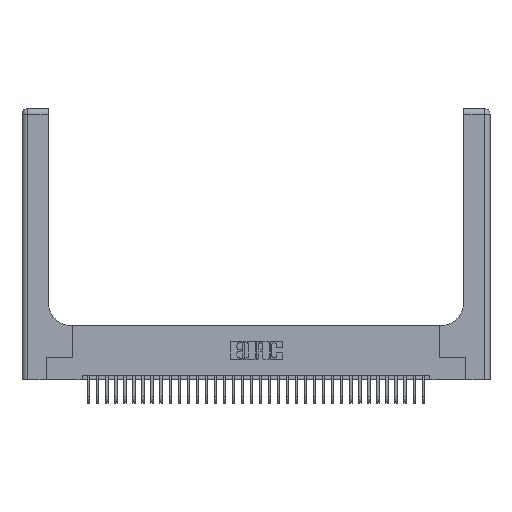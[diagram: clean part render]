
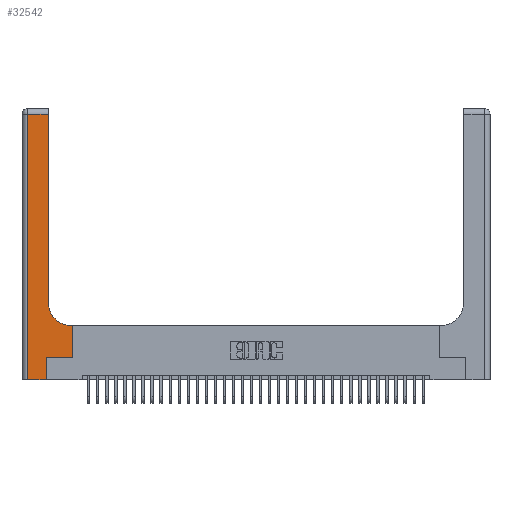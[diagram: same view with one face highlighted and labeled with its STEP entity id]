
A CAD part, top view. The second image highlights one B-rep face of the part: STEP entity #32542.
In plain terms, the highlighted planar face has unit normal (0, 0, 1).
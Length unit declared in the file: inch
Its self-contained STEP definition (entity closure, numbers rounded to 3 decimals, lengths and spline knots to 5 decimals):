
#166 = DIRECTION ( 'NONE',  ( 0., -1., 0. ) ) ;
#376 = VERTEX_POINT ( 'NONE', #32147 ) ;
#468 = CIRCLE ( 'NONE', #10036, 0.25 ) ;
#1016 = VERTEX_POINT ( 'NONE', #6161 ) ;
#1091 = CARTESIAN_POINT ( 'NONE',  ( 0., 3., 0.37 ) ) ;
#1142 = ORIENTED_EDGE ( 'NONE', *, *, #17522, .T. ) ;
#2170 = CARTESIAN_POINT ( 'NONE',  ( 0.5585, 0.25, 0.37 ) ) ;
#2455 = ORIENTED_EDGE ( 'NONE', *, *, #17761, .T. ) ;
#2585 = LINE ( 'NONE', #32829, #16213 ) ;
#3007 = EDGE_CURVE ( 'NONE', #6427, #1016, #31712, .T. ) ;
#3385 = VECTOR ( 'NONE', #26445, 39.37008 ) ;
#3393 = CARTESIAN_POINT ( 'NONE',  ( 0.2915, 0.6, 0.37 ) ) ;
#3431 = ORIENTED_EDGE ( 'NONE', *, *, #26476, .T. ) ;
#3520 = VERTEX_POINT ( 'NONE', #12462 ) ;
#4020 = VERTEX_POINT ( 'NONE', #26422 ) ;
#4056 = ORIENTED_EDGE ( 'NONE', *, *, #34689, .T. ) ;
#4371 = VERTEX_POINT ( 'NONE', #27849 ) ;
#4481 = CARTESIAN_POINT ( 'NONE',  ( 0.5585, 0.25, 0.37 ) ) ;
#4905 = VECTOR ( 'NONE', #166, 39.37008 ) ;
#5585 = CARTESIAN_POINT ( 'NONE',  ( 0.2915, 0.85, 0.37 ) ) ;
#6161 = CARTESIAN_POINT ( 'NONE',  ( 0.5585, 0.6, 0.37 ) ) ;
#6427 = VERTEX_POINT ( 'NONE', #2170 ) ;
#7512 = VERTEX_POINT ( 'NONE', #18950 ) ;
#8931 = VECTOR ( 'NONE', #18878, 39.37008 ) ;
#9338 = DIRECTION ( 'NONE',  ( 0., 1., 0. ) ) ;
#10036 = AXIS2_PLACEMENT_3D ( 'NONE', #34138, #17114, #37005 ) ;
#10242 = LINE ( 'NONE', #3393, #3385 ) ;
#10463 = CARTESIAN_POINT ( 'NONE',  ( 0., 0., 0.37 ) ) ;
#11689 = VECTOR ( 'NONE', #15035, 39.37008 ) ;
#12445 = CARTESIAN_POINT ( 'NONE',  ( 0.06, 2.94, 0.37 ) ) ;
#12462 = CARTESIAN_POINT ( 'NONE',  ( 0.269, 0., 0.37 ) ) ;
#12748 = VERTEX_POINT ( 'NONE', #5585 ) ;
#13800 = LINE ( 'NONE', #10463, #33816 ) ;
#13873 = LINE ( 'NONE', #34886, #35668 ) ;
#15035 = DIRECTION ( 'NONE',  ( 1., 0., 0. ) ) ;
#15732 = DIRECTION ( 'NONE',  ( -1., 0., 0. ) ) ;
#16213 = VECTOR ( 'NONE', #35671, 39.37008 ) ;
#17114 = DIRECTION ( 'NONE',  ( 0., 0., -1. ) ) ;
#17227 = CARTESIAN_POINT ( 'NONE',  ( 0.06, 3., 0.37 ) ) ;
#17522 = EDGE_CURVE ( 'NONE', #3520, #7512, #27700, .T. ) ;
#17761 = EDGE_CURVE ( 'NONE', #12748, #4020, #13873, .T. ) ;
#18509 = VERTEX_POINT ( 'NONE', #12445 ) ;
#18878 = DIRECTION ( 'NONE',  ( 0., 1., 0. ) ) ;
#18950 = CARTESIAN_POINT ( 'NONE',  ( 0.269, 0.25, 0.37 ) ) ;
#19938 = EDGE_CURVE ( 'NONE', #1016, #4371, #10242, .T. ) ;
#19995 = ORIENTED_EDGE ( 'NONE', *, *, #36030, .T. ) ;
#20140 = VECTOR ( 'NONE', #25517, 39.37008 ) ;
#20658 = CARTESIAN_POINT ( 'NONE',  ( 0.269, 0.25, 0.37 ) ) ;
#20813 = EDGE_CURVE ( 'NONE', #376, #3520, #13800, .T. ) ;
#22586 = ORIENTED_EDGE ( 'NONE', *, *, #20813, .T. ) ;
#22629 = CARTESIAN_POINT ( 'NONE',  ( 0.269, 0., 0.37 ) ) ;
#22778 = AXIS2_PLACEMENT_3D ( 'NONE', #1091, #32775, #15732 ) ;
#24768 = DIRECTION ( 'NONE',  ( 1., 0., 0. ) ) ;
#25517 = DIRECTION ( 'NONE',  ( 0., 1., 0. ) ) ;
#26019 = LINE ( 'NONE', #20658, #11689 ) ;
#26422 = CARTESIAN_POINT ( 'NONE',  ( 0.2915, 2.94, 0.37 ) ) ;
#26445 = DIRECTION ( 'NONE',  ( -1., 0., 0. ) ) ;
#26476 = EDGE_CURVE ( 'NONE', #18509, #376, #35349, .T. ) ;
#27084 = PLANE ( 'NONE',  #22778 ) ;
#27700 = LINE ( 'NONE', #22629, #20140 ) ;
#27849 = CARTESIAN_POINT ( 'NONE',  ( 0.5415, 0.6, 0.37 ) ) ;
#30524 = ORIENTED_EDGE ( 'NONE', *, *, #32204, .T. ) ;
#31712 = LINE ( 'NONE', #4481, #8931 ) ;
#32147 = CARTESIAN_POINT ( 'NONE',  ( 0.06, 0., 0.37 ) ) ;
#32204 = EDGE_CURVE ( 'NONE', #4371, #12748, #468, .T. ) ;
#32423 = ORIENTED_EDGE ( 'NONE', *, *, #19938, .T. ) ;
#32542 = ADVANCED_FACE ( 'NONE', ( #32848 ), #27084, .F. ) ;
#32775 = DIRECTION ( 'NONE',  ( 0., 0., -1. ) ) ;
#32829 = CARTESIAN_POINT ( 'NONE',  ( 0., 2.94, 0.37 ) ) ;
#32848 = FACE_OUTER_BOUND ( 'NONE', #37204, .T. ) ;
#33816 = VECTOR ( 'NONE', #24768, 39.37008 ) ;
#34138 = CARTESIAN_POINT ( 'NONE',  ( 0.5415, 0.85, 0.37 ) ) ;
#34689 = EDGE_CURVE ( 'NONE', #4020, #18509, #2585, .T. ) ;
#34886 = CARTESIAN_POINT ( 'NONE',  ( 0.2915, 3., 0.37 ) ) ;
#35349 = LINE ( 'NONE', #17227, #4905 ) ;
#35668 = VECTOR ( 'NONE', #9338, 39.37008 ) ;
#35671 = DIRECTION ( 'NONE',  ( -1., 0., 0. ) ) ;
#36030 = EDGE_CURVE ( 'NONE', #7512, #6427, #26019, .T. ) ;
#37005 = DIRECTION ( 'NONE',  ( 1., 0., 0. ) ) ;
#37038 = ORIENTED_EDGE ( 'NONE', *, *, #3007, .T. ) ;
#37204 = EDGE_LOOP ( 'NONE', ( #2455, #4056, #3431, #22586, #1142, #19995, #37038, #32423, #30524 ) ) ;
